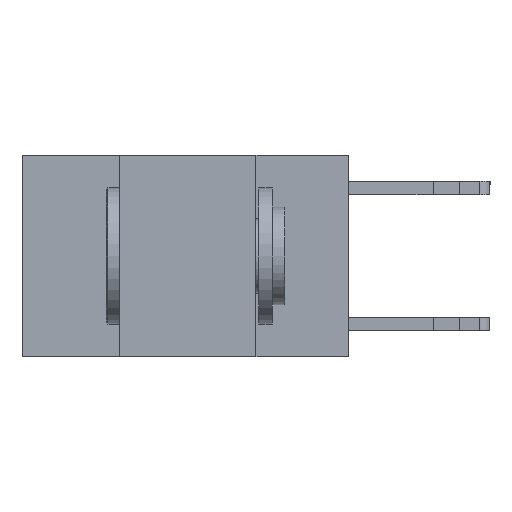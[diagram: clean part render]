
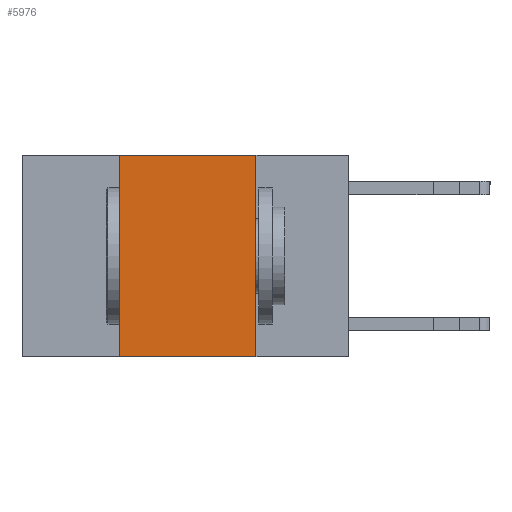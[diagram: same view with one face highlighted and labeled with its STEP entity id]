
A CAD part, left-side view. The second image highlights one B-rep face of the part: STEP entity #5976.
In plain terms, the highlighted planar face has unit normal (-1, 0, 0).
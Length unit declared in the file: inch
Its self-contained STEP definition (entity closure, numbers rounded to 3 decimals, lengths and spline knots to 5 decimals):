
#500 = ORIENTED_EDGE ( 'NONE', *, *, #12462, .F. ) ;
#515 = CARTESIAN_POINT ( 'NONE',  ( 0., 0.6, 0. ) ) ;
#1420 = CARTESIAN_POINT ( 'NONE',  ( 0., 0.6, -0.37 ) ) ;
#2326 = EDGE_CURVE ( 'NONE', #10652, #7640, #4955, .T. ) ;
#2447 = FACE_OUTER_BOUND ( 'NONE', #4661, .T. ) ;
#2734 = VECTOR ( 'NONE', #8276, 39.37008 ) ;
#2747 = CARTESIAN_POINT ( 'NONE',  ( 0., 0.42, -0.37 ) ) ;
#3187 = ORIENTED_EDGE ( 'NONE', *, *, #6499, .T. ) ;
#3343 = VERTEX_POINT ( 'NONE', #10708 ) ;
#3805 = VECTOR ( 'NONE', #11784, 39.37008 ) ;
#4229 = VECTOR ( 'NONE', #12046, 39.37008 ) ;
#4582 = DIRECTION ( 'NONE',  ( 1., 0., 0. ) ) ;
#4606 = ORIENTED_EDGE ( 'NONE', *, *, #2326, .F. ) ;
#4661 = EDGE_LOOP ( 'NONE', ( #4606, #8380, #500, #3187 ) ) ;
#4955 = LINE ( 'NONE', #8009, #4229 ) ;
#5065 = AXIS2_PLACEMENT_3D ( 'NONE', #515, #4582, #8558 ) ;
#5525 = CARTESIAN_POINT ( 'NONE',  ( 0., 0.42, 0. ) ) ;
#5976 = ADVANCED_FACE ( 'NONE', ( #2447 ), #6424, .F. ) ;
#6393 = LINE ( 'NONE', #5525, #6640 ) ;
#6424 = PLANE ( 'NONE',  #5065 ) ;
#6499 = EDGE_CURVE ( 'NONE', #11394, #7640, #10516, .T. ) ;
#6572 = EDGE_CURVE ( 'NONE', #3343, #10652, #7600, .T. ) ;
#6640 = VECTOR ( 'NONE', #10706, 39.37008 ) ;
#7600 = LINE ( 'NONE', #11655, #3805 ) ;
#7640 = VERTEX_POINT ( 'NONE', #9351 ) ;
#8009 = CARTESIAN_POINT ( 'NONE',  ( 0., 0.17, 0. ) ) ;
#8276 = DIRECTION ( 'NONE',  ( 0., -1., 0. ) ) ;
#8380 = ORIENTED_EDGE ( 'NONE', *, *, #6572, .F. ) ;
#8558 = DIRECTION ( 'NONE',  ( 0., 0., -1. ) ) ;
#9290 = CARTESIAN_POINT ( 'NONE',  ( 0., 0.17, 0. ) ) ;
#9351 = CARTESIAN_POINT ( 'NONE',  ( 0., 0.17, -0.37 ) ) ;
#10516 = LINE ( 'NONE', #1420, #2734 ) ;
#10652 = VERTEX_POINT ( 'NONE', #9290 ) ;
#10706 = DIRECTION ( 'NONE',  ( 0., 0., 1. ) ) ;
#10708 = CARTESIAN_POINT ( 'NONE',  ( 0., 0.42, 0. ) ) ;
#11394 = VERTEX_POINT ( 'NONE', #2747 ) ;
#11655 = CARTESIAN_POINT ( 'NONE',  ( 0., 0.6, 0. ) ) ;
#11784 = DIRECTION ( 'NONE',  ( 0., -1., 0. ) ) ;
#12046 = DIRECTION ( 'NONE',  ( 0., 0., -1. ) ) ;
#12462 = EDGE_CURVE ( 'NONE', #11394, #3343, #6393, .T. ) ;
